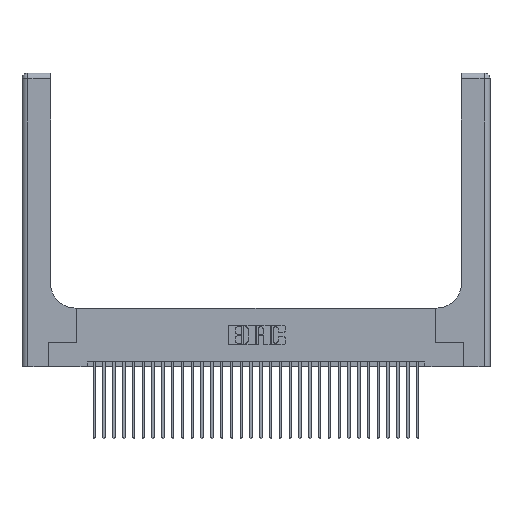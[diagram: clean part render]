
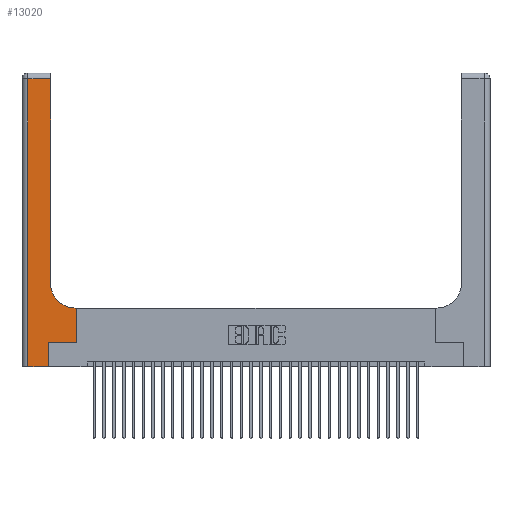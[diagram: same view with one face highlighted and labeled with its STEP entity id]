
A CAD part, top view. The second image highlights one B-rep face of the part: STEP entity #13020.
In plain terms, the highlighted planar face has unit normal (0, 0, 1).
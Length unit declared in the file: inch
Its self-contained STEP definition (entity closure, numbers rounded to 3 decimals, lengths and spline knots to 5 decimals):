
#1343 = VECTOR ( 'NONE', #7376, 39.37008 ) ;
#2083 = CARTESIAN_POINT ( 'NONE',  ( 0.5585, 0.25, 0.37 ) ) ;
#2112 = EDGE_CURVE ( 'NONE', #3625, #22938, #13710, .T. ) ;
#2872 = CARTESIAN_POINT ( 'NONE',  ( 0.5415, 0.85, 0.37 ) ) ;
#3335 = CARTESIAN_POINT ( 'NONE',  ( 0., 3., 0.37 ) ) ;
#3446 = PLANE ( 'NONE',  #32137 ) ;
#3625 = VERTEX_POINT ( 'NONE', #19719 ) ;
#3675 = DIRECTION ( 'NONE',  ( 1., 0., 0. ) ) ;
#3919 = DIRECTION ( 'NONE',  ( 0., 1., 0. ) ) ;
#4271 = EDGE_CURVE ( 'NONE', #22938, #10342, #7262, .T. ) ;
#4348 = LINE ( 'NONE', #13665, #11190 ) ;
#4756 = DIRECTION ( 'NONE',  ( 0., 1., 0. ) ) ;
#5318 = CARTESIAN_POINT ( 'NONE',  ( 0.269, 0.25, 0.37 ) ) ;
#5511 = DIRECTION ( 'NONE',  ( 1., 0., 0. ) ) ;
#6100 = DIRECTION ( 'NONE',  ( -1., 0., 0. ) ) ;
#6918 = LINE ( 'NONE', #2083, #26228 ) ;
#7100 = EDGE_CURVE ( 'NONE', #20819, #23795, #6918, .T. ) ;
#7262 = LINE ( 'NONE', #17429, #13954 ) ;
#7346 = EDGE_CURVE ( 'NONE', #31975, #23269, #14011, .T. ) ;
#7376 = DIRECTION ( 'NONE',  ( -1., 0., 0. ) ) ;
#7378 = LINE ( 'NONE', #13967, #27462 ) ;
#7392 = DIRECTION ( 'NONE',  ( 0., 1., 0. ) ) ;
#8122 = VECTOR ( 'NONE', #18207, 39.37008 ) ;
#9192 = VERTEX_POINT ( 'NONE', #25752 ) ;
#9411 = ORIENTED_EDGE ( 'NONE', *, *, #25430, .T. ) ;
#10342 = VERTEX_POINT ( 'NONE', #24922 ) ;
#11173 = ORIENTED_EDGE ( 'NONE', *, *, #2112, .T. ) ;
#11190 = VECTOR ( 'NONE', #21242, 39.37008 ) ;
#12540 = LINE ( 'NONE', #5318, #13318 ) ;
#13020 = ADVANCED_FACE ( 'NONE', ( #21871 ), #3446, .F. ) ;
#13318 = VECTOR ( 'NONE', #20484, 39.37008 ) ;
#13665 = CARTESIAN_POINT ( 'NONE',  ( 0.06, 3., 0.37 ) ) ;
#13710 = CIRCLE ( 'NONE', #29647, 0.25 ) ;
#13954 = VECTOR ( 'NONE', #4756, 39.37008 ) ;
#13967 = CARTESIAN_POINT ( 'NONE',  ( 0., 0., 0.37 ) ) ;
#14011 = LINE ( 'NONE', #31690, #26603 ) ;
#14830 = LINE ( 'NONE', #15704, #8122 ) ;
#15036 = LINE ( 'NONE', #22446, #1343 ) ;
#15704 = CARTESIAN_POINT ( 'NONE',  ( 0.2915, 0.6, 0.37 ) ) ;
#15919 = CARTESIAN_POINT ( 'NONE',  ( 0.269, 0.25, 0.37 ) ) ;
#16852 = CARTESIAN_POINT ( 'NONE',  ( 0.5585, 0.25, 0.37 ) ) ;
#17060 = ORIENTED_EDGE ( 'NONE', *, *, #18081, .T. ) ;
#17429 = CARTESIAN_POINT ( 'NONE',  ( 0.2915, 3., 0.37 ) ) ;
#17967 = CARTESIAN_POINT ( 'NONE',  ( 0.5585, 0.6, 0.37 ) ) ;
#18081 = EDGE_CURVE ( 'NONE', #9192, #29888, #4348, .T. ) ;
#18207 = DIRECTION ( 'NONE',  ( -1., 0., 0. ) ) ;
#19189 = ORIENTED_EDGE ( 'NONE', *, *, #23210, .T. ) ;
#19719 = CARTESIAN_POINT ( 'NONE',  ( 0.5415, 0.6, 0.37 ) ) ;
#20484 = DIRECTION ( 'NONE',  ( 1., 0., 0. ) ) ;
#20666 = DIRECTION ( 'NONE',  ( 0., 0., -1. ) ) ;
#20819 = VERTEX_POINT ( 'NONE', #16852 ) ;
#20959 = CARTESIAN_POINT ( 'NONE',  ( 0.06, 0., 0.37 ) ) ;
#21221 = DIRECTION ( 'NONE',  ( 0., 0., -1. ) ) ;
#21242 = DIRECTION ( 'NONE',  ( 0., -1., 0. ) ) ;
#21310 = ORIENTED_EDGE ( 'NONE', *, *, #4271, .T. ) ;
#21698 = CARTESIAN_POINT ( 'NONE',  ( 0.269, 0., 0.37 ) ) ;
#21871 = FACE_OUTER_BOUND ( 'NONE', #27764, .T. ) ;
#22446 = CARTESIAN_POINT ( 'NONE',  ( 0., 2.94, 0.37 ) ) ;
#22741 = EDGE_CURVE ( 'NONE', #29888, #31975, #7378, .T. ) ;
#22938 = VERTEX_POINT ( 'NONE', #24732 ) ;
#23210 = EDGE_CURVE ( 'NONE', #23795, #3625, #14830, .T. ) ;
#23269 = VERTEX_POINT ( 'NONE', #15919 ) ;
#23795 = VERTEX_POINT ( 'NONE', #17967 ) ;
#24001 = ORIENTED_EDGE ( 'NONE', *, *, #29243, .T. ) ;
#24732 = CARTESIAN_POINT ( 'NONE',  ( 0.2915, 0.85, 0.37 ) ) ;
#24789 = ORIENTED_EDGE ( 'NONE', *, *, #22741, .T. ) ;
#24922 = CARTESIAN_POINT ( 'NONE',  ( 0.2915, 2.94, 0.37 ) ) ;
#25430 = EDGE_CURVE ( 'NONE', #23269, #20819, #12540, .T. ) ;
#25752 = CARTESIAN_POINT ( 'NONE',  ( 0.06, 2.94, 0.37 ) ) ;
#26228 = VECTOR ( 'NONE', #7392, 39.37008 ) ;
#26603 = VECTOR ( 'NONE', #3919, 39.37008 ) ;
#26878 = ORIENTED_EDGE ( 'NONE', *, *, #7346, .T. ) ;
#27462 = VECTOR ( 'NONE', #3675, 39.37008 ) ;
#27764 = EDGE_LOOP ( 'NONE', ( #21310, #24001, #17060, #24789, #26878, #9411, #29306, #19189, #11173 ) ) ;
#29243 = EDGE_CURVE ( 'NONE', #10342, #9192, #15036, .T. ) ;
#29306 = ORIENTED_EDGE ( 'NONE', *, *, #7100, .T. ) ;
#29647 = AXIS2_PLACEMENT_3D ( 'NONE', #2872, #20666, #5511 ) ;
#29888 = VERTEX_POINT ( 'NONE', #20959 ) ;
#31690 = CARTESIAN_POINT ( 'NONE',  ( 0.269, 0., 0.37 ) ) ;
#31975 = VERTEX_POINT ( 'NONE', #21698 ) ;
#32137 = AXIS2_PLACEMENT_3D ( 'NONE', #3335, #21221, #6100 ) ;
